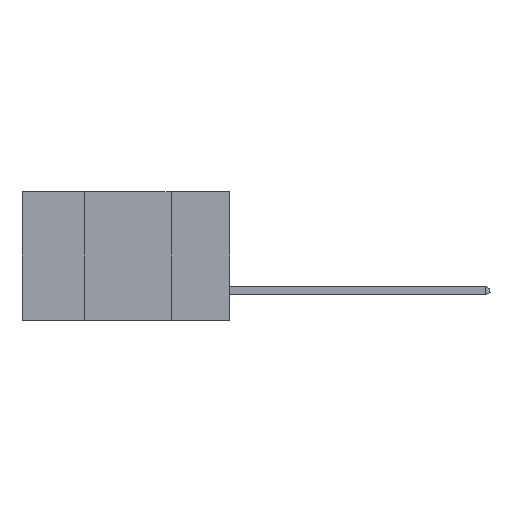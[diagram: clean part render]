
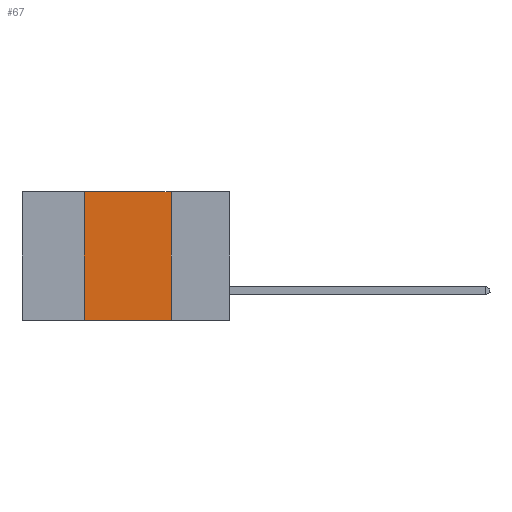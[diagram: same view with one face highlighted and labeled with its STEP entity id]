
A CAD part, left-side view. The second image highlights one B-rep face of the part: STEP entity #67.
In plain terms, the highlighted planar face has unit normal (-1, 0, 0).
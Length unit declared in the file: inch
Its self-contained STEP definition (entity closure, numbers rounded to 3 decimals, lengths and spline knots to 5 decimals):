
#67 = ADVANCED_FACE ( 'NONE', ( #7938 ), #24219, .F. ) ;
#705 = ORIENTED_EDGE ( 'NONE', *, *, #21580, .F. ) ;
#1668 = VERTEX_POINT ( 'NONE', #29084 ) ;
#1901 = LINE ( 'NONE', #6218, #26425 ) ;
#2415 = VERTEX_POINT ( 'NONE', #19423 ) ;
#2714 = ORIENTED_EDGE ( 'NONE', *, *, #28404, .T. ) ;
#6218 = CARTESIAN_POINT ( 'NONE',  ( 0., 0.17, 0. ) ) ;
#6569 = LINE ( 'NONE', #21157, #7317 ) ;
#6600 = LINE ( 'NONE', #17585, #10333 ) ;
#7317 = VECTOR ( 'NONE', #9645, 39.37008 ) ;
#7624 = DIRECTION ( 'NONE',  ( 0., 0., 1. ) ) ;
#7938 = FACE_OUTER_BOUND ( 'NONE', #18978, .T. ) ;
#8161 = ORIENTED_EDGE ( 'NONE', *, *, #26318, .F. ) ;
#8736 = AXIS2_PLACEMENT_3D ( 'NONE', #28877, #14641, #12480 ) ;
#9645 = DIRECTION ( 'NONE',  ( 0., -1., 0. ) ) ;
#10333 = VECTOR ( 'NONE', #7624, 39.37008 ) ;
#12323 = DIRECTION ( 'NONE',  ( 0., -1., 0. ) ) ;
#12480 = DIRECTION ( 'NONE',  ( 0., 0., -1. ) ) ;
#13151 = VERTEX_POINT ( 'NONE', #26386 ) ;
#14641 = DIRECTION ( 'NONE',  ( 1., 0., 0. ) ) ;
#14811 = CARTESIAN_POINT ( 'NONE',  ( 0., 0.42, -0.37 ) ) ;
#16965 = CARTESIAN_POINT ( 'NONE',  ( 0., 0.6, 0. ) ) ;
#17585 = CARTESIAN_POINT ( 'NONE',  ( 0., 0.42, 0. ) ) ;
#18035 = LINE ( 'NONE', #16965, #25505 ) ;
#18816 = ORIENTED_EDGE ( 'NONE', *, *, #24719, .F. ) ;
#18978 = EDGE_LOOP ( 'NONE', ( #705, #8161, #18816, #2714 ) ) ;
#19423 = CARTESIAN_POINT ( 'NONE',  ( 0., 0.17, 0. ) ) ;
#21063 = DIRECTION ( 'NONE',  ( 0., 0., -1. ) ) ;
#21157 = CARTESIAN_POINT ( 'NONE',  ( 0., 0.6, -0.37 ) ) ;
#21580 = EDGE_CURVE ( 'NONE', #2415, #13151, #1901, .T. ) ;
#24219 = PLANE ( 'NONE',  #8736 ) ;
#24719 = EDGE_CURVE ( 'NONE', #26634, #1668, #6600, .T. ) ;
#25505 = VECTOR ( 'NONE', #12323, 39.37008 ) ;
#26318 = EDGE_CURVE ( 'NONE', #1668, #2415, #18035, .T. ) ;
#26386 = CARTESIAN_POINT ( 'NONE',  ( 0., 0.17, -0.37 ) ) ;
#26425 = VECTOR ( 'NONE', #21063, 39.37008 ) ;
#26634 = VERTEX_POINT ( 'NONE', #14811 ) ;
#28404 = EDGE_CURVE ( 'NONE', #26634, #13151, #6569, .T. ) ;
#28877 = CARTESIAN_POINT ( 'NONE',  ( 0., 0.6, 0. ) ) ;
#29084 = CARTESIAN_POINT ( 'NONE',  ( 0., 0.42, 0. ) ) ;
